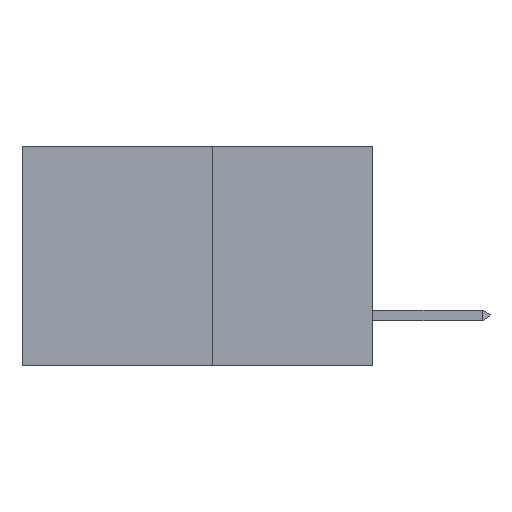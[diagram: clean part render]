
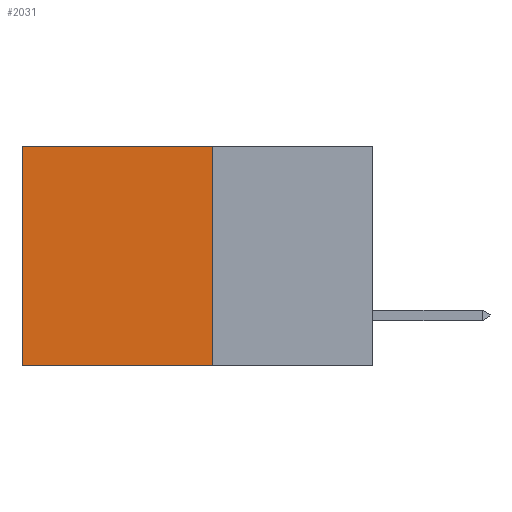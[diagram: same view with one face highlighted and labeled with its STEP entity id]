
A CAD part, left-side view. The second image highlights one B-rep face of the part: STEP entity #2031.
In plain terms, the highlighted planar face has unit normal (-1, 0, 0).
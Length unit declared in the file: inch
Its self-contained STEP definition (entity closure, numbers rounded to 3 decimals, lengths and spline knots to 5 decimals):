
#329 = CARTESIAN_POINT ( 'NONE',  ( 0.277, 0.27, 0. ) ) ;
#457 = VECTOR ( 'NONE', #2754, 39.37008 ) ;
#1059 = CARTESIAN_POINT ( 'NONE',  ( 0.277, 0.27, -0.37 ) ) ;
#1597 = ORIENTED_EDGE ( 'NONE', *, *, #10124, .T. ) ;
#2031 = ADVANCED_FACE ( 'NONE', ( #4646 ), #7490, .F. ) ;
#2054 = DIRECTION ( 'NONE',  ( 0., 0., -1. ) ) ;
#2113 = VECTOR ( 'NONE', #3325, 39.37008 ) ;
#2274 = ORIENTED_EDGE ( 'NONE', *, *, #6814, .F. ) ;
#2418 = DIRECTION ( 'NONE',  ( 1., 0., 0. ) ) ;
#2641 = VECTOR ( 'NONE', #2054, 39.37008 ) ;
#2678 = ORIENTED_EDGE ( 'NONE', *, *, #10628, .T. ) ;
#2754 = DIRECTION ( 'NONE',  ( 0., 1., 0. ) ) ;
#2913 = EDGE_LOOP ( 'NONE', ( #1597, #3226, #2274, #2678 ) ) ;
#3124 = VERTEX_POINT ( 'NONE', #10056 ) ;
#3226 = ORIENTED_EDGE ( 'NONE', *, *, #9550, .F. ) ;
#3325 = DIRECTION ( 'NONE',  ( 0., 1., 0. ) ) ;
#4210 = VECTOR ( 'NONE', #7692, 39.37008 ) ;
#4646 = FACE_OUTER_BOUND ( 'NONE', #2913, .T. ) ;
#5255 = LINE ( 'NONE', #1059, #2641 ) ;
#5310 = AXIS2_PLACEMENT_3D ( 'NONE', #10867, #2418, #8909 ) ;
#5630 = CARTESIAN_POINT ( 'NONE',  ( 0.277, 0.59, 0. ) ) ;
#6300 = VERTEX_POINT ( 'NONE', #9830 ) ;
#6517 = LINE ( 'NONE', #10050, #4210 ) ;
#6814 = EDGE_CURVE ( 'NONE', #10496, #6300, #5255, .T. ) ;
#7058 = CARTESIAN_POINT ( 'NONE',  ( 0.277, 0.27, -0.37 ) ) ;
#7490 = PLANE ( 'NONE',  #5310 ) ;
#7692 = DIRECTION ( 'NONE',  ( 0., 0., -1. ) ) ;
#8909 = DIRECTION ( 'NONE',  ( 0., 0., -1. ) ) ;
#8945 = LINE ( 'NONE', #10010, #2113 ) ;
#9550 = EDGE_CURVE ( 'NONE', #6300, #3124, #9716, .T. ) ;
#9716 = LINE ( 'NONE', #7058, #457 ) ;
#9796 = VERTEX_POINT ( 'NONE', #5630 ) ;
#9830 = CARTESIAN_POINT ( 'NONE',  ( 0.277, 0.27, -0.37 ) ) ;
#10010 = CARTESIAN_POINT ( 'NONE',  ( 0.277, 0.27, 0. ) ) ;
#10050 = CARTESIAN_POINT ( 'NONE',  ( 0.277, 0.59, -0.37 ) ) ;
#10056 = CARTESIAN_POINT ( 'NONE',  ( 0.277, 0.59, -0.37 ) ) ;
#10124 = EDGE_CURVE ( 'NONE', #9796, #3124, #6517, .T. ) ;
#10496 = VERTEX_POINT ( 'NONE', #329 ) ;
#10628 = EDGE_CURVE ( 'NONE', #10496, #9796, #8945, .T. ) ;
#10867 = CARTESIAN_POINT ( 'NONE',  ( 0.277, 0.27, -0.37 ) ) ;
